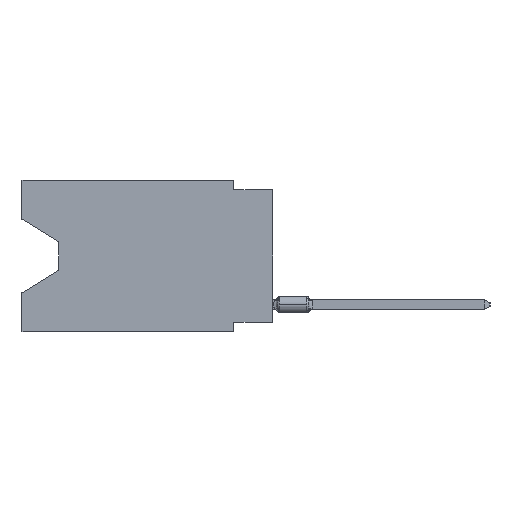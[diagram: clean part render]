
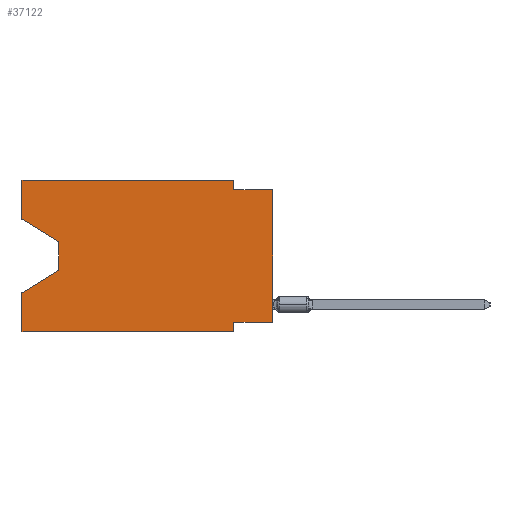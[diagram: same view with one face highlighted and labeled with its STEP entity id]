
A CAD part, left-side view. The second image highlights one B-rep face of the part: STEP entity #37122.
In plain terms, the highlighted planar face has unit normal (-1, 0, 0).
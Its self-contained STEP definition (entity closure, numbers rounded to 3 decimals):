
#301 = VECTOR ( 'NONE', #29756, 1000. ) ;
#489 = FACE_OUTER_BOUND ( 'NONE', #71956, .T. ) ;
#532 = CARTESIAN_POINT ( 'NONE',  ( 0., 16.383, 0. ) ) ;
#669 = VECTOR ( 'NONE', #54337, 1000. ) ;
#864 = EDGE_CURVE ( 'NONE', #65940, #51698, #48737, .T. ) ;
#1485 = VECTOR ( 'NONE', #29666, 1000. ) ;
#1894 = DIRECTION ( 'NONE',  ( 0., 0., 1. ) ) ;
#2254 = DIRECTION ( 'NONE',  ( 0., 1., 0. ) ) ;
#2654 = CARTESIAN_POINT ( 'NONE',  ( 0., 13.97, -4.013 ) ) ;
#2788 = ORIENTED_EDGE ( 'NONE', *, *, #76326, .F. ) ;
#4923 = ORIENTED_EDGE ( 'NONE', *, *, #7106, .T. ) ;
#5294 = PLANE ( 'NONE',  #24454 ) ;
#5641 = ORIENTED_EDGE ( 'NONE', *, *, #17710, .F. ) ;
#5754 = EDGE_CURVE ( 'NONE', #21754, #10737, #17777, .T. ) ;
#5806 = VERTEX_POINT ( 'NONE', #41206 ) ;
#6154 = CARTESIAN_POINT ( 'NONE',  ( 0., 2.54, 0. ) ) ;
#7106 = EDGE_CURVE ( 'NONE', #31213, #21754, #24138, .T. ) ;
#7966 = VERTEX_POINT ( 'NONE', #19451 ) ;
#8032 = VERTEX_POINT ( 'NONE', #22971 ) ;
#9673 = CARTESIAN_POINT ( 'NONE',  ( 0., 0., -0.635 ) ) ;
#9852 = VECTOR ( 'NONE', #29581, 1000. ) ;
#10737 = VERTEX_POINT ( 'NONE', #66320 ) ;
#11822 = CARTESIAN_POINT ( 'NONE',  ( 0., 13.97, -5.893 ) ) ;
#12427 = CARTESIAN_POINT ( 'NONE',  ( 0., 16.383, 0. ) ) ;
#13765 = CARTESIAN_POINT ( 'NONE',  ( 0., 16.383, 0. ) ) ;
#15998 = VERTEX_POINT ( 'NONE', #46781 ) ;
#17257 = VECTOR ( 'NONE', #24498, 1000. ) ;
#17387 = DIRECTION ( 'NONE',  ( 0., 0., -1. ) ) ;
#17710 = EDGE_CURVE ( 'NONE', #15998, #49878, #54680, .T. ) ;
#17777 = LINE ( 'NONE', #11822, #1485 ) ;
#19448 = DIRECTION ( 'NONE',  ( 0., -1., 0. ) ) ;
#19451 = CARTESIAN_POINT ( 'NONE',  ( 0., 0., -9.271 ) ) ;
#19711 = CARTESIAN_POINT ( 'NONE',  ( 0., 16.383, -2.546 ) ) ;
#19864 = CARTESIAN_POINT ( 'NONE',  ( 0., 2.54, -0.635 ) ) ;
#20128 = EDGE_CURVE ( 'NONE', #8032, #51698, #73472, .T. ) ;
#20136 = LINE ( 'NONE', #62634, #44162 ) ;
#20357 = VECTOR ( 'NONE', #54555, 1000. ) ;
#21754 = VERTEX_POINT ( 'NONE', #46734 ) ;
#22971 = CARTESIAN_POINT ( 'NONE',  ( 0., 16.383, -9.906 ) ) ;
#24138 = LINE ( 'NONE', #72986, #63563 ) ;
#24454 = AXIS2_PLACEMENT_3D ( 'NONE', #12427, #49338, #48953 ) ;
#24498 = DIRECTION ( 'NONE',  ( 0., 0., 1. ) ) ;
#25310 = ORIENTED_EDGE ( 'NONE', *, *, #69368, .F. ) ;
#27531 = LINE ( 'NONE', #45043, #43661 ) ;
#29581 = DIRECTION ( 'NONE',  ( 0., 0., -1. ) ) ;
#29666 = DIRECTION ( 'NONE',  ( 0., 0.855, -0.519 ) ) ;
#29756 = DIRECTION ( 'NONE',  ( 0., -0.855, -0.519 ) ) ;
#30316 = LINE ( 'NONE', #532, #20357 ) ;
#31213 = VERTEX_POINT ( 'NONE', #2654 ) ;
#32460 = LINE ( 'NONE', #45569, #50698 ) ;
#34002 = EDGE_CURVE ( 'NONE', #7966, #69241, #47600, .T. ) ;
#35285 = VECTOR ( 'NONE', #19448, 1000. ) ;
#35437 = ORIENTED_EDGE ( 'NONE', *, *, #34002, .T. ) ;
#36193 = VERTEX_POINT ( 'NONE', #19864 ) ;
#36703 = ORIENTED_EDGE ( 'NONE', *, *, #864, .F. ) ;
#37122 = ADVANCED_FACE ( 'NONE', ( #489 ), #5294, .F. ) ;
#41206 = CARTESIAN_POINT ( 'NONE',  ( 0., 2.54, 0. ) ) ;
#43018 = EDGE_CURVE ( 'NONE', #5806, #36193, #66142, .T. ) ;
#43661 = VECTOR ( 'NONE', #69255, 1000. ) ;
#44162 = VECTOR ( 'NONE', #2254, 1000. ) ;
#44686 = EDGE_CURVE ( 'NONE', #7966, #65940, #20136, .T. ) ;
#45043 = CARTESIAN_POINT ( 'NONE',  ( 0., 0., -0.635 ) ) ;
#45569 = CARTESIAN_POINT ( 'NONE',  ( 0., 16.383, 0. ) ) ;
#46734 = CARTESIAN_POINT ( 'NONE',  ( 0., 13.97, -5.893 ) ) ;
#46781 = CARTESIAN_POINT ( 'NONE',  ( 0., 16.383, -2.546 ) ) ;
#47600 = LINE ( 'NONE', #59507, #669 ) ;
#48737 = LINE ( 'NONE', #78150, #72980 ) ;
#48953 = DIRECTION ( 'NONE',  ( 0., 0., -1. ) ) ;
#49338 = DIRECTION ( 'NONE',  ( 1., 0., 0. ) ) ;
#49878 = VERTEX_POINT ( 'NONE', #67353 ) ;
#50028 = CARTESIAN_POINT ( 'NONE',  ( 0., 2.54, -9.271 ) ) ;
#50548 = CARTESIAN_POINT ( 'NONE',  ( 0., 2.54, -9.906 ) ) ;
#50698 = VECTOR ( 'NONE', #1894, 1000. ) ;
#51698 = VERTEX_POINT ( 'NONE', #50548 ) ;
#54337 = DIRECTION ( 'NONE',  ( 0., 0., 1. ) ) ;
#54555 = DIRECTION ( 'NONE',  ( 0., -1., 0. ) ) ;
#54680 = LINE ( 'NONE', #13765, #17257 ) ;
#57984 = ORIENTED_EDGE ( 'NONE', *, *, #43018, .F. ) ;
#59507 = CARTESIAN_POINT ( 'NONE',  ( 0., 0., 0. ) ) ;
#59684 = ORIENTED_EDGE ( 'NONE', *, *, #70048, .F. ) ;
#62634 = CARTESIAN_POINT ( 'NONE',  ( 0., 0., -9.271 ) ) ;
#63563 = VECTOR ( 'NONE', #72589, 1000. ) ;
#63699 = ORIENTED_EDGE ( 'NONE', *, *, #44686, .F. ) ;
#65940 = VERTEX_POINT ( 'NONE', #50028 ) ;
#66142 = LINE ( 'NONE', #6154, #9852 ) ;
#66320 = CARTESIAN_POINT ( 'NONE',  ( 0., 16.383, -7.36 ) ) ;
#66345 = CARTESIAN_POINT ( 'NONE',  ( 0., 16.383, -9.906 ) ) ;
#67353 = CARTESIAN_POINT ( 'NONE',  ( 0., 16.383, 0. ) ) ;
#69241 = VERTEX_POINT ( 'NONE', #9673 ) ;
#69255 = DIRECTION ( 'NONE',  ( 0., -1., 0. ) ) ;
#69368 = EDGE_CURVE ( 'NONE', #8032, #10737, #32460, .T. ) ;
#70048 = EDGE_CURVE ( 'NONE', #49878, #5806, #30316, .T. ) ;
#71956 = EDGE_LOOP ( 'NONE', ( #72751, #4923, #72699, #25310, #78489, #36703, #63699, #35437, #2788, #57984, #59684, #5641 ) ) ;
#72125 = EDGE_CURVE ( 'NONE', #15998, #31213, #74126, .T. ) ;
#72589 = DIRECTION ( 'NONE',  ( 0., 0., -1. ) ) ;
#72699 = ORIENTED_EDGE ( 'NONE', *, *, #5754, .T. ) ;
#72751 = ORIENTED_EDGE ( 'NONE', *, *, #72125, .T. ) ;
#72980 = VECTOR ( 'NONE', #17387, 1000. ) ;
#72986 = CARTESIAN_POINT ( 'NONE',  ( 0., 13.97, -4.013 ) ) ;
#73472 = LINE ( 'NONE', #66345, #35285 ) ;
#74126 = LINE ( 'NONE', #19711, #301 ) ;
#76326 = EDGE_CURVE ( 'NONE', #36193, #69241, #27531, .T. ) ;
#78150 = CARTESIAN_POINT ( 'NONE',  ( 0., 2.54, -9.906 ) ) ;
#78489 = ORIENTED_EDGE ( 'NONE', *, *, #20128, .T. ) ;
